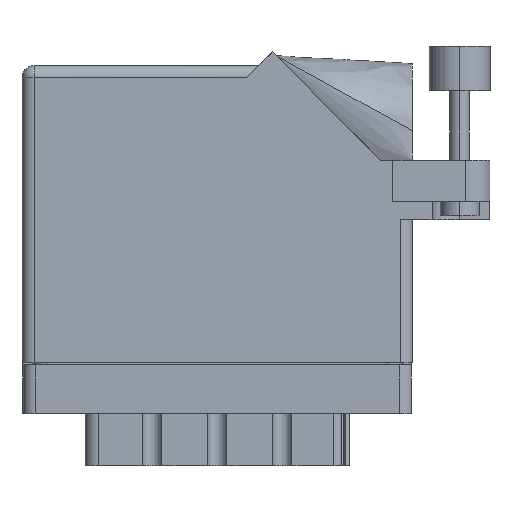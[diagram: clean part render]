
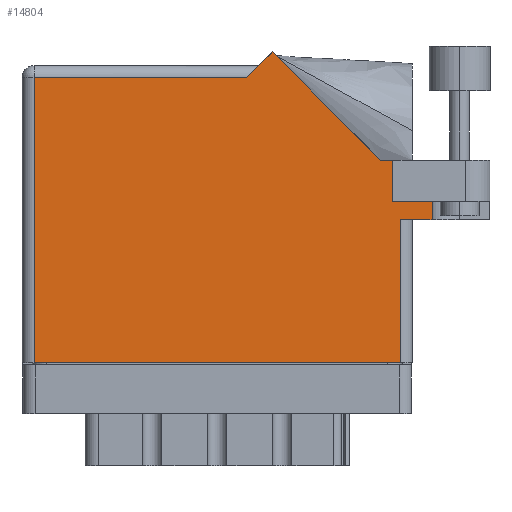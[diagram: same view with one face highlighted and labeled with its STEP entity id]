
A CAD part, front view. The second image highlights one B-rep face of the part: STEP entity #14804.
In plain terms, the highlighted face is planar.
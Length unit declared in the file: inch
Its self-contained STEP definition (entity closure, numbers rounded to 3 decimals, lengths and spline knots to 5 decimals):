
#132 = LINE ( 'NONE', #23821, #26932 ) ;
#592 = CARTESIAN_POINT ( 'NONE',  ( 1.155, 1.468, 0. ) ) ;
#831 = VERTEX_POINT ( 'NONE', #33946 ) ;
#1598 = EDGE_CURVE ( 'NONE', #14533, #14368, #36325, .T. ) ;
#1770 = ORIENTED_EDGE ( 'NONE', *, *, #5692, .T. ) ;
#2029 = ORIENTED_EDGE ( 'NONE', *, *, #1598, .T. ) ;
#2163 = DIRECTION ( 'NONE',  ( 1., 0., 0. ) ) ;
#2972 = VECTOR ( 'NONE', #2163, 39.37008 ) ;
#3701 = DIRECTION ( 'NONE',  ( 0., -1., 0. ) ) ;
#3975 = CARTESIAN_POINT ( 'NONE',  ( 2.1115, 1.16177, 0. ) ) ;
#5331 = LINE ( 'NONE', #16925, #11777 ) ;
#5603 = EDGE_CURVE ( 'NONE', #21224, #17798, #14267, .T. ) ;
#5692 = EDGE_CURVE ( 'NONE', #17798, #831, #15390, .T. ) ;
#5754 = LINE ( 'NONE', #3975, #32210 ) ;
#6261 = DIRECTION ( 'NONE',  ( 1., 0., 0. ) ) ;
#6525 = CARTESIAN_POINT ( 'NONE',  ( 2.1115, 0.831, 0. ) ) ;
#6534 = VECTOR ( 'NONE', #6261, 39.37008 ) ;
#7174 = EDGE_CURVE ( 'NONE', #831, #17678, #132, .T. ) ;
#7493 = CARTESIAN_POINT ( 'NONE',  ( 0.062, 0., 0. ) ) ;
#7718 = LINE ( 'NONE', #25180, #25983 ) ;
#8034 = EDGE_CURVE ( 'NONE', #26096, #35040, #5331, .T. ) ;
#8461 = ORIENTED_EDGE ( 'NONE', *, *, #31986, .T. ) ;
#8886 = EDGE_LOOP ( 'NONE', ( #13697, #13217, #27066, #31263, #13684, #29982, #1770, #18493, #27798, #8461, #2029 ) ) ;
#9008 = CARTESIAN_POINT ( 'NONE',  ( 1.217, 1.53, 0. ) ) ;
#10107 = EDGE_CURVE ( 'NONE', #14368, #26096, #7718, .T. ) ;
#10520 = EDGE_CURVE ( 'NONE', #35040, #34493, #28179, .T. ) ;
#11777 = VECTOR ( 'NONE', #28494, 39.37008 ) ;
#11977 = LINE ( 'NONE', #29794, #6534 ) ;
#12535 = DIRECTION ( 'NONE',  ( 0., -1., 0. ) ) ;
#13152 = LINE ( 'NONE', #21343, #24146 ) ;
#13217 = ORIENTED_EDGE ( 'NONE', *, *, #8034, .T. ) ;
#13255 = PLANE ( 'NONE',  #37105 ) ;
#13684 = ORIENTED_EDGE ( 'NONE', *, *, #17499, .F. ) ;
#13697 = ORIENTED_EDGE ( 'NONE', *, *, #10107, .T. ) ;
#13825 = VECTOR ( 'NONE', #3701, 39.37008 ) ;
#14267 = LINE ( 'NONE', #28879, #23066 ) ;
#14368 = VERTEX_POINT ( 'NONE', #29805 ) ;
#14441 = CARTESIAN_POINT ( 'NONE',  ( 1.948, 0., 0. ) ) ;
#14533 = VERTEX_POINT ( 'NONE', #14759 ) ;
#14759 = CARTESIAN_POINT ( 'NONE',  ( 0.062, 1.468, 0. ) ) ;
#14804 = ADVANCED_FACE ( 'NONE', ( #22558 ), #13255, .F. ) ;
#15197 = DIRECTION ( 'NONE',  ( -1., 0., 0. ) ) ;
#15286 = DIRECTION ( 'NONE',  ( -0.707, 0.707, 0. ) ) ;
#15390 = LINE ( 'NONE', #35114, #33208 ) ;
#15463 = LINE ( 'NONE', #9008, #34098 ) ;
#15552 = EDGE_CURVE ( 'NONE', #17678, #24349, #15463, .T. ) ;
#16866 = CARTESIAN_POINT ( 'NONE',  ( 1.91, 1.044, 0. ) ) ;
#16925 = CARTESIAN_POINT ( 'NONE',  ( 1.948, 0.737, 0. ) ) ;
#17499 = EDGE_CURVE ( 'NONE', #21224, #29518, #11977, .T. ) ;
#17678 = VERTEX_POINT ( 'NONE', #33742 ) ;
#17798 = VERTEX_POINT ( 'NONE', #16866 ) ;
#17980 = CARTESIAN_POINT ( 'NONE',  ( 2.1115, 0.737, 0. ) ) ;
#18493 = ORIENTED_EDGE ( 'NONE', *, *, #7174, .T. ) ;
#19146 = CARTESIAN_POINT ( 'NONE',  ( 0., 1.53, 0. ) ) ;
#20978 = EDGE_CURVE ( 'NONE', #29518, #34493, #5754, .T. ) ;
#21153 = DIRECTION ( 'NONE',  ( -1., 0., 0. ) ) ;
#21224 = VERTEX_POINT ( 'NONE', #34316 ) ;
#21343 = CARTESIAN_POINT ( 'NONE',  ( 0., 1.468, 0. ) ) ;
#22558 = FACE_OUTER_BOUND ( 'NONE', #8886, .T. ) ;
#22999 = DIRECTION ( 'NONE',  ( 0., 1., 0. ) ) ;
#23066 = VECTOR ( 'NONE', #22999, 39.37008 ) ;
#23821 = CARTESIAN_POINT ( 'NONE',  ( 1.84442, 1.044, 0. ) ) ;
#24146 = VECTOR ( 'NONE', #21153, 39.37008 ) ;
#24349 = VERTEX_POINT ( 'NONE', #592 ) ;
#25180 = CARTESIAN_POINT ( 'NONE',  ( 0., 0., 0. ) ) ;
#25983 = VECTOR ( 'NONE', #36752, 39.37008 ) ;
#26096 = VERTEX_POINT ( 'NONE', #14441 ) ;
#26526 = CARTESIAN_POINT ( 'NONE',  ( 1.948, 0.737, 0. ) ) ;
#26932 = VECTOR ( 'NONE', #15286, 39.37008 ) ;
#27032 = DIRECTION ( 'NONE',  ( -0.707, -0.707, 0. ) ) ;
#27066 = ORIENTED_EDGE ( 'NONE', *, *, #10520, .T. ) ;
#27797 = CARTESIAN_POINT ( 'NONE',  ( 2.01, 0.737, 0. ) ) ;
#27798 = ORIENTED_EDGE ( 'NONE', *, *, #15552, .T. ) ;
#28179 = LINE ( 'NONE', #27797, #2972 ) ;
#28494 = DIRECTION ( 'NONE',  ( 0., 1., 0. ) ) ;
#28879 = CARTESIAN_POINT ( 'NONE',  ( 1.91, 0.831, 0. ) ) ;
#29518 = VERTEX_POINT ( 'NONE', #6525 ) ;
#29794 = CARTESIAN_POINT ( 'NONE',  ( 1.91, 0.831, 0. ) ) ;
#29805 = CARTESIAN_POINT ( 'NONE',  ( 0.062, 0., 0. ) ) ;
#29982 = ORIENTED_EDGE ( 'NONE', *, *, #5603, .T. ) ;
#30710 = DIRECTION ( 'NONE',  ( -1., 0., 0. ) ) ;
#31263 = ORIENTED_EDGE ( 'NONE', *, *, #20978, .F. ) ;
#31986 = EDGE_CURVE ( 'NONE', #24349, #14533, #13152, .T. ) ;
#32210 = VECTOR ( 'NONE', #12535, 39.37008 ) ;
#33208 = VECTOR ( 'NONE', #15197, 39.37008 ) ;
#33742 = CARTESIAN_POINT ( 'NONE',  ( 1.28771, 1.60071, 0. ) ) ;
#33917 = DIRECTION ( 'NONE',  ( 0., 0., -1. ) ) ;
#33946 = CARTESIAN_POINT ( 'NONE',  ( 1.84442, 1.044, 0. ) ) ;
#34098 = VECTOR ( 'NONE', #27032, 39.37008 ) ;
#34316 = CARTESIAN_POINT ( 'NONE',  ( 1.91, 0.831, 0. ) ) ;
#34493 = VERTEX_POINT ( 'NONE', #17980 ) ;
#35040 = VERTEX_POINT ( 'NONE', #26526 ) ;
#35114 = CARTESIAN_POINT ( 'NONE',  ( 2.41, 1.044, 0. ) ) ;
#36325 = LINE ( 'NONE', #7493, #13825 ) ;
#36752 = DIRECTION ( 'NONE',  ( 1., 0., 0. ) ) ;
#37105 = AXIS2_PLACEMENT_3D ( 'NONE', #19146, #33917, #30710 ) ;
